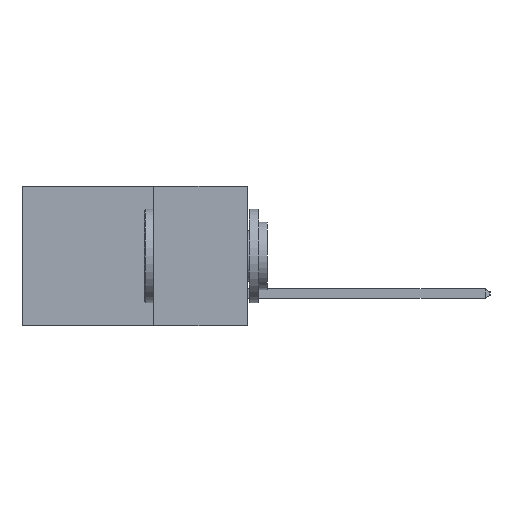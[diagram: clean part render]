
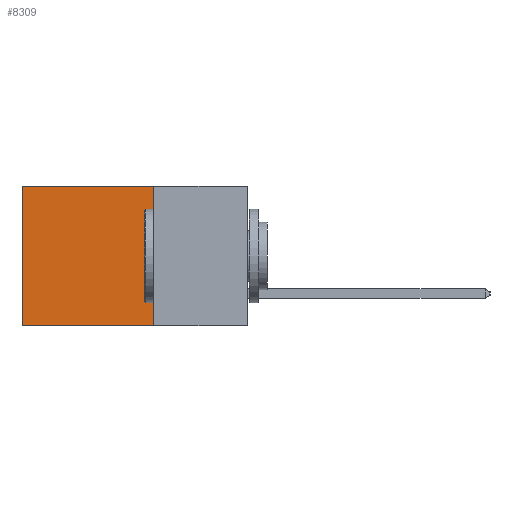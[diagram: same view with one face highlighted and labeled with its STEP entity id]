
A CAD part, left-side view. The second image highlights one B-rep face of the part: STEP entity #8309.
In plain terms, the highlighted planar face has unit normal (-1, 0, 0).
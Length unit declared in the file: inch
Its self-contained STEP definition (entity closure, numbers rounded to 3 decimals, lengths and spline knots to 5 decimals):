
#77 = CARTESIAN_POINT ( 'NONE',  ( 0.298, 0.6, 0. ) ) ;
#933 = VERTEX_POINT ( 'NONE', #6405 ) ;
#1764 = DIRECTION ( 'NONE',  ( 0., 0., -1. ) ) ;
#1853 = LINE ( 'NONE', #8859, #11660 ) ;
#1877 = DIRECTION ( 'NONE',  ( 0., 1., 0. ) ) ;
#1921 = VERTEX_POINT ( 'NONE', #77 ) ;
#2087 = DIRECTION ( 'NONE',  ( 0., 1., 0. ) ) ;
#2330 = FACE_OUTER_BOUND ( 'NONE', #4834, .T. ) ;
#2450 = DIRECTION ( 'NONE',  ( 0., 0., -1. ) ) ;
#2475 = EDGE_CURVE ( 'NONE', #3910, #8243, #8466, .T. ) ;
#2689 = VECTOR ( 'NONE', #2450, 39.37008 ) ;
#2870 = CARTESIAN_POINT ( 'NONE',  ( 0.298, 0.25, 0. ) ) ;
#3341 = CARTESIAN_POINT ( 'NONE',  ( 0.298, 0.6, 0. ) ) ;
#3744 = LINE ( 'NONE', #3892, #10695 ) ;
#3892 = CARTESIAN_POINT ( 'NONE',  ( 0.298, 0.25, 0. ) ) ;
#3910 = VERTEX_POINT ( 'NONE', #2870 ) ;
#4265 = ORIENTED_EDGE ( 'NONE', *, *, #5323, .T. ) ;
#4514 = ORIENTED_EDGE ( 'NONE', *, *, #8578, .F. ) ;
#4834 = EDGE_LOOP ( 'NONE', ( #4265, #4514, #5019, #6236 ) ) ;
#5019 = ORIENTED_EDGE ( 'NONE', *, *, #2475, .F. ) ;
#5323 = EDGE_CURVE ( 'NONE', #1921, #933, #6877, .T. ) ;
#6236 = ORIENTED_EDGE ( 'NONE', *, *, #8441, .T. ) ;
#6405 = CARTESIAN_POINT ( 'NONE',  ( 0.298, 0.6, -0.37 ) ) ;
#6499 = AXIS2_PLACEMENT_3D ( 'NONE', #7072, #7320, #7299 ) ;
#6829 = CARTESIAN_POINT ( 'NONE',  ( 0.298, 0.25, 0. ) ) ;
#6877 = LINE ( 'NONE', #3341, #9317 ) ;
#6905 = PLANE ( 'NONE',  #6499 ) ;
#7072 = CARTESIAN_POINT ( 'NONE',  ( 0.298, 0.25, 0. ) ) ;
#7299 = DIRECTION ( 'NONE',  ( 0., 0., -1. ) ) ;
#7320 = DIRECTION ( 'NONE',  ( 1., 0., 0. ) ) ;
#8243 = VERTEX_POINT ( 'NONE', #9878 ) ;
#8309 = ADVANCED_FACE ( 'NONE', ( #2330 ), #6905, .F. ) ;
#8441 = EDGE_CURVE ( 'NONE', #3910, #1921, #3744, .T. ) ;
#8466 = LINE ( 'NONE', #6829, #2689 ) ;
#8578 = EDGE_CURVE ( 'NONE', #8243, #933, #1853, .T. ) ;
#8859 = CARTESIAN_POINT ( 'NONE',  ( 0.298, 0.25, -0.37 ) ) ;
#9317 = VECTOR ( 'NONE', #1764, 39.37008 ) ;
#9878 = CARTESIAN_POINT ( 'NONE',  ( 0.298, 0.25, -0.37 ) ) ;
#10695 = VECTOR ( 'NONE', #1877, 39.37008 ) ;
#11660 = VECTOR ( 'NONE', #2087, 39.37008 ) ;
